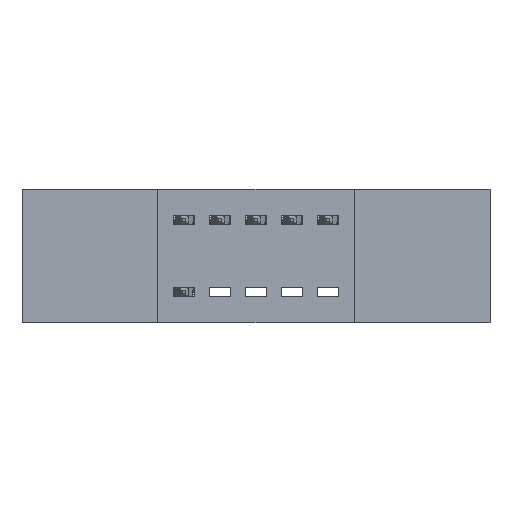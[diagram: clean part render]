
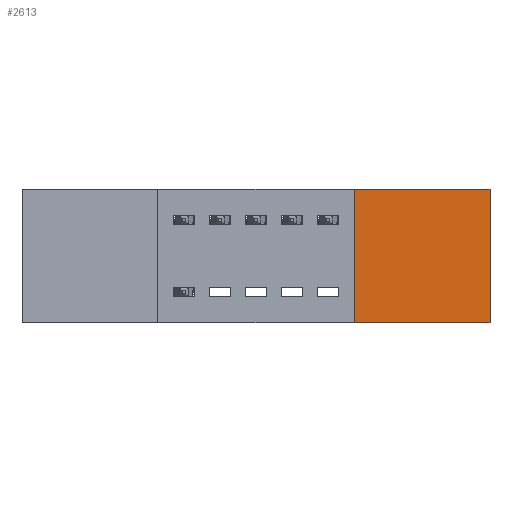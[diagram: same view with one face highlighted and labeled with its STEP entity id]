
A CAD part, front view. The second image highlights one B-rep face of the part: STEP entity #2613.
In plain terms, the highlighted planar face has unit normal (0, -1, 0).
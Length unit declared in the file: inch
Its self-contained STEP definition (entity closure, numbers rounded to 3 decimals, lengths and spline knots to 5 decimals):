
#210 = AXIS2_PLACEMENT_3D ( 'NONE', #4523, #5733, #7200 ) ;
#329 = VECTOR ( 'NONE', #1645, 39.37008 ) ;
#576 = LINE ( 'NONE', #2787, #5433 ) ;
#630 = EDGE_CURVE ( 'NONE', #954, #6641, #5351, .T. ) ;
#741 = ORIENTED_EDGE ( 'NONE', *, *, #1836, .F. ) ;
#836 = ORIENTED_EDGE ( 'NONE', *, *, #630, .F. ) ;
#954 = VERTEX_POINT ( 'NONE', #4089 ) ;
#1123 = CARTESIAN_POINT ( 'NONE',  ( 0.923, 0., -0.37 ) ) ;
#1429 = PLANE ( 'NONE',  #210 ) ;
#1645 = DIRECTION ( 'NONE',  ( -1., 0., 0. ) ) ;
#1836 = EDGE_CURVE ( 'NONE', #6849, #954, #576, .T. ) ;
#1998 = VECTOR ( 'NONE', #2135, 39.37008 ) ;
#2135 = DIRECTION ( 'NONE',  ( 0., 0., -1. ) ) ;
#2189 = CARTESIAN_POINT ( 'NONE',  ( 0., 0., -0.37 ) ) ;
#2613 = ADVANCED_FACE ( 'NONE', ( #4638 ), #1429, .T. ) ;
#2639 = EDGE_CURVE ( 'NONE', #3416, #6849, #2749, .T. ) ;
#2726 = CARTESIAN_POINT ( 'NONE',  ( 0.923, 0., -0.37 ) ) ;
#2749 = LINE ( 'NONE', #2726, #5856 ) ;
#2787 = CARTESIAN_POINT ( 'NONE',  ( 0., 0., 0. ) ) ;
#3158 = EDGE_LOOP ( 'NONE', ( #4112, #5050, #836, #741 ) ) ;
#3238 = CARTESIAN_POINT ( 'NONE',  ( 0.923, 0., 0. ) ) ;
#3416 = VERTEX_POINT ( 'NONE', #1123 ) ;
#3454 = EDGE_CURVE ( 'NONE', #6641, #3416, #3718, .T. ) ;
#3718 = LINE ( 'NONE', #2189, #329 ) ;
#4089 = CARTESIAN_POINT ( 'NONE',  ( 1.3, 0., 0. ) ) ;
#4112 = ORIENTED_EDGE ( 'NONE', *, *, #2639, .F. ) ;
#4201 = DIRECTION ( 'NONE',  ( 0., 0., 1. ) ) ;
#4498 = CARTESIAN_POINT ( 'NONE',  ( 1.3, 0., 0. ) ) ;
#4523 = CARTESIAN_POINT ( 'NONE',  ( 0., 0., -0.37 ) ) ;
#4638 = FACE_OUTER_BOUND ( 'NONE', #3158, .T. ) ;
#5050 = ORIENTED_EDGE ( 'NONE', *, *, #3454, .F. ) ;
#5252 = CARTESIAN_POINT ( 'NONE',  ( 1.3, 0., -0.37 ) ) ;
#5351 = LINE ( 'NONE', #4498, #1998 ) ;
#5433 = VECTOR ( 'NONE', #7597, 39.37008 ) ;
#5733 = DIRECTION ( 'NONE',  ( 0., -1., 0. ) ) ;
#5856 = VECTOR ( 'NONE', #4201, 39.37008 ) ;
#6641 = VERTEX_POINT ( 'NONE', #5252 ) ;
#6849 = VERTEX_POINT ( 'NONE', #3238 ) ;
#7200 = DIRECTION ( 'NONE',  ( 0., 0., -1. ) ) ;
#7597 = DIRECTION ( 'NONE',  ( 1., 0., 0. ) ) ;
